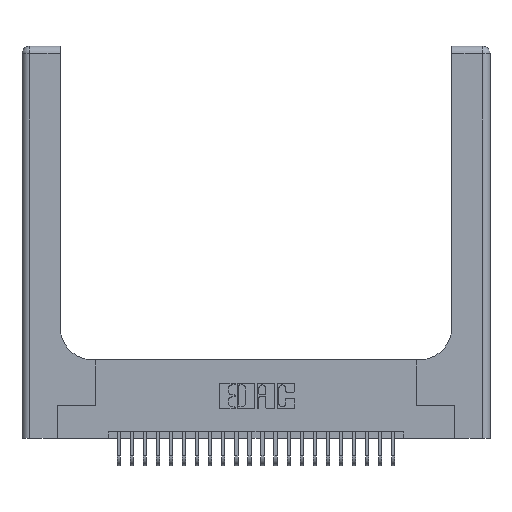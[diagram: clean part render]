
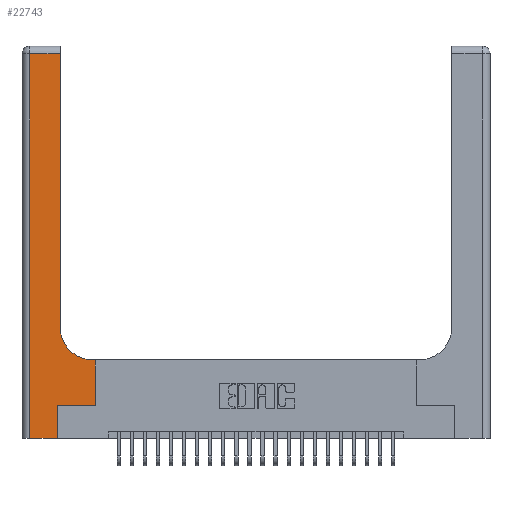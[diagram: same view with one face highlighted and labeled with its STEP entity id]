
A CAD part, top view. The second image highlights one B-rep face of the part: STEP entity #22743.
In plain terms, the highlighted planar face has unit normal (0, 0, 1).
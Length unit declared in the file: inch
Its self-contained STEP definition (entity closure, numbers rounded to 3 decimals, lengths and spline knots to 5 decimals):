
#640 = DIRECTION ( 'NONE',  ( 1., 0., 0. ) ) ;
#1304 = DIRECTION ( 'NONE',  ( 0., 1., 0. ) ) ;
#1561 = ORIENTED_EDGE ( 'NONE', *, *, #18531, .T. ) ;
#2382 = DIRECTION ( 'NONE',  ( -1., 0., 0. ) ) ;
#3207 = LINE ( 'NONE', #17336, #23915 ) ;
#3560 = DIRECTION ( 'NONE',  ( -1., 0., 0. ) ) ;
#3584 = ORIENTED_EDGE ( 'NONE', *, *, #11008, .T. ) ;
#3899 = EDGE_CURVE ( 'NONE', #17659, #10141, #4152, .T. ) ;
#3932 = VECTOR ( 'NONE', #3560, 39.37008 ) ;
#4152 = CIRCLE ( 'NONE', #18121, 0.25 ) ;
#4641 = VERTEX_POINT ( 'NONE', #22051 ) ;
#5619 = VERTEX_POINT ( 'NONE', #8661 ) ;
#5815 = CARTESIAN_POINT ( 'NONE',  ( 0.5585, 0.25, 0.37 ) ) ;
#5976 = VECTOR ( 'NONE', #20611, 39.37008 ) ;
#6197 = ORIENTED_EDGE ( 'NONE', *, *, #3899, .T. ) ;
#6430 = CARTESIAN_POINT ( 'NONE',  ( 0.2915, 0.6, 0.37 ) ) ;
#6895 = DIRECTION ( 'NONE',  ( 0., 0., -1. ) ) ;
#7172 = ORIENTED_EDGE ( 'NONE', *, *, #23597, .T. ) ;
#7292 = CARTESIAN_POINT ( 'NONE',  ( 0.2915, 3., 0.37 ) ) ;
#7490 = EDGE_CURVE ( 'NONE', #22697, #16686, #22475, .T. ) ;
#7523 = VECTOR ( 'NONE', #1304, 39.37008 ) ;
#8661 = CARTESIAN_POINT ( 'NONE',  ( 0.06, 2.94, 0.37 ) ) ;
#9421 = CARTESIAN_POINT ( 'NONE',  ( 0.5415, 0.85, 0.37 ) ) ;
#10141 = VERTEX_POINT ( 'NONE', #14503 ) ;
#11008 = EDGE_CURVE ( 'NONE', #16686, #17032, #3207, .T. ) ;
#11515 = DIRECTION ( 'NONE',  ( 1., 0., 0. ) ) ;
#12040 = VECTOR ( 'NONE', #16311, 39.37008 ) ;
#12307 = CARTESIAN_POINT ( 'NONE',  ( 0.2915, 2.94, 0.37 ) ) ;
#12392 = CARTESIAN_POINT ( 'NONE',  ( 0., 0., 0.37 ) ) ;
#12712 = LINE ( 'NONE', #16224, #12040 ) ;
#13145 = LINE ( 'NONE', #19999, #7523 ) ;
#13438 = ORIENTED_EDGE ( 'NONE', *, *, #16407, .T. ) ;
#13587 = EDGE_CURVE ( 'NONE', #17032, #14867, #13145, .T. ) ;
#13643 = DIRECTION ( 'NONE',  ( 0., 1., 0. ) ) ;
#13909 = CARTESIAN_POINT ( 'NONE',  ( 0., 2.94, 0.37 ) ) ;
#14503 = CARTESIAN_POINT ( 'NONE',  ( 0.2915, 0.85, 0.37 ) ) ;
#14814 = VERTEX_POINT ( 'NONE', #12307 ) ;
#14867 = VERTEX_POINT ( 'NONE', #24716 ) ;
#15201 = PLANE ( 'NONE',  #24472 ) ;
#15783 = LINE ( 'NONE', #7292, #20580 ) ;
#15981 = ORIENTED_EDGE ( 'NONE', *, *, #17694, .T. ) ;
#16224 = CARTESIAN_POINT ( 'NONE',  ( 0.06, 3., 0.37 ) ) ;
#16311 = DIRECTION ( 'NONE',  ( 0., -1., 0. ) ) ;
#16407 = EDGE_CURVE ( 'NONE', #5619, #4641, #12712, .T. ) ;
#16686 = VERTEX_POINT ( 'NONE', #17406 ) ;
#17032 = VERTEX_POINT ( 'NONE', #5815 ) ;
#17336 = CARTESIAN_POINT ( 'NONE',  ( 0.269, 0.25, 0.37 ) ) ;
#17406 = CARTESIAN_POINT ( 'NONE',  ( 0.269, 0.25, 0.37 ) ) ;
#17659 = VERTEX_POINT ( 'NONE', #24920 ) ;
#17694 = EDGE_CURVE ( 'NONE', #14867, #17659, #20008, .T. ) ;
#18121 = AXIS2_PLACEMENT_3D ( 'NONE', #9421, #23790, #11515 ) ;
#18531 = EDGE_CURVE ( 'NONE', #10141, #14814, #15783, .T. ) ;
#18582 = CARTESIAN_POINT ( 'NONE',  ( 0.269, 0., 0.37 ) ) ;
#18778 = EDGE_LOOP ( 'NONE', ( #1561, #7172, #13438, #24282, #19536, #3584, #26180, #15981, #6197 ) ) ;
#19171 = CARTESIAN_POINT ( 'NONE',  ( 0.269, 0., 0.37 ) ) ;
#19343 = CARTESIAN_POINT ( 'NONE',  ( 0., 3., 0.37 ) ) ;
#19375 = VECTOR ( 'NONE', #2382, 39.37008 ) ;
#19536 = ORIENTED_EDGE ( 'NONE', *, *, #7490, .T. ) ;
#19999 = CARTESIAN_POINT ( 'NONE',  ( 0.5585, 0.25, 0.37 ) ) ;
#20008 = LINE ( 'NONE', #6430, #19375 ) ;
#20483 = LINE ( 'NONE', #13909, #3932 ) ;
#20580 = VECTOR ( 'NONE', #13643, 39.37008 ) ;
#20611 = DIRECTION ( 'NONE',  ( 0., 1., 0. ) ) ;
#20622 = DIRECTION ( 'NONE',  ( 1., 0., 0. ) ) ;
#21394 = DIRECTION ( 'NONE',  ( -1., 0., 0. ) ) ;
#22051 = CARTESIAN_POINT ( 'NONE',  ( 0.06, 0., 0.37 ) ) ;
#22475 = LINE ( 'NONE', #18582, #5976 ) ;
#22697 = VERTEX_POINT ( 'NONE', #19171 ) ;
#22743 = ADVANCED_FACE ( 'NONE', ( #22745 ), #15201, .F. ) ;
#22745 = FACE_OUTER_BOUND ( 'NONE', #18778, .T. ) ;
#23597 = EDGE_CURVE ( 'NONE', #14814, #5619, #20483, .T. ) ;
#23790 = DIRECTION ( 'NONE',  ( 0., 0., -1. ) ) ;
#23915 = VECTOR ( 'NONE', #640, 39.37008 ) ;
#24282 = ORIENTED_EDGE ( 'NONE', *, *, #26018, .T. ) ;
#24472 = AXIS2_PLACEMENT_3D ( 'NONE', #19343, #6895, #21394 ) ;
#24716 = CARTESIAN_POINT ( 'NONE',  ( 0.5585, 0.6, 0.37 ) ) ;
#24920 = CARTESIAN_POINT ( 'NONE',  ( 0.5415, 0.6, 0.37 ) ) ;
#25047 = VECTOR ( 'NONE', #20622, 39.37008 ) ;
#25692 = LINE ( 'NONE', #12392, #25047 ) ;
#26018 = EDGE_CURVE ( 'NONE', #4641, #22697, #25692, .T. ) ;
#26180 = ORIENTED_EDGE ( 'NONE', *, *, #13587, .T. ) ;
